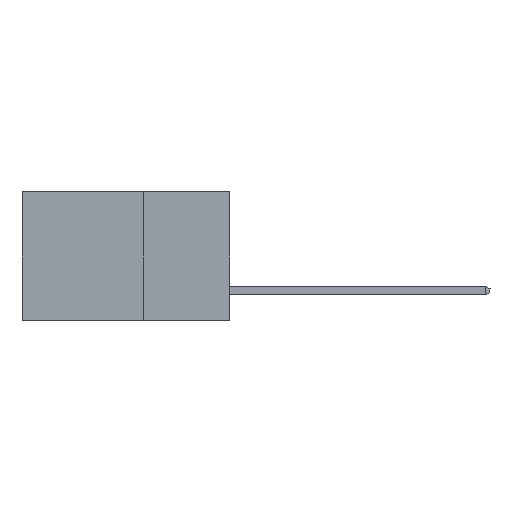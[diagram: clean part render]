
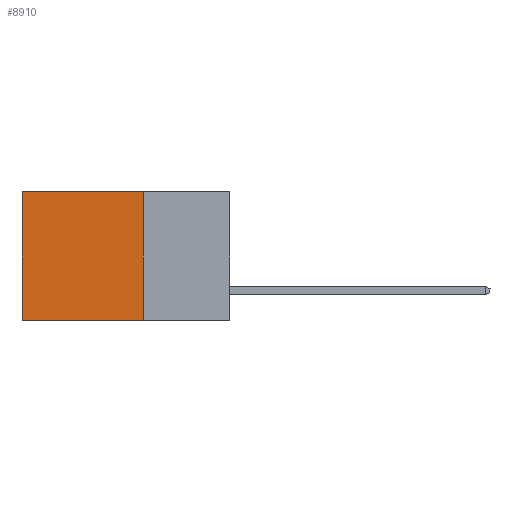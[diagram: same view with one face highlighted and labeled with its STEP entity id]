
A CAD part, left-side view. The second image highlights one B-rep face of the part: STEP entity #8910.
In plain terms, the highlighted planar face has unit normal (-1, 0, 0).
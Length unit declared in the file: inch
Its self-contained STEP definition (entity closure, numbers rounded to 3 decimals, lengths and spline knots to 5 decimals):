
#572 = CARTESIAN_POINT ( 'NONE',  ( 0.2615, 0.6, -0.37 ) ) ;
#685 = VERTEX_POINT ( 'NONE', #4246 ) ;
#836 = CARTESIAN_POINT ( 'NONE',  ( 0.2615, 0.25, -0.37 ) ) ;
#913 = EDGE_CURVE ( 'NONE', #2880, #7285, #18450, .T. ) ;
#2241 = EDGE_LOOP ( 'NONE', ( #13702, #8557, #10275, #5009 ) ) ;
#2442 = CARTESIAN_POINT ( 'NONE',  ( 0.2615, 0.25, 0. ) ) ;
#2776 = CARTESIAN_POINT ( 'NONE',  ( 0.2615, 0.25, -0.37 ) ) ;
#2880 = VERTEX_POINT ( 'NONE', #4384 ) ;
#3271 = VECTOR ( 'NONE', #8469, 39.37008 ) ;
#3718 = DIRECTION ( 'NONE',  ( 1., 0., 0. ) ) ;
#4246 = CARTESIAN_POINT ( 'NONE',  ( 0.2615, 0.25, 0. ) ) ;
#4384 = CARTESIAN_POINT ( 'NONE',  ( 0.2615, 0.6, 0. ) ) ;
#4489 = CARTESIAN_POINT ( 'NONE',  ( 0.2615, 0.25, -0.37 ) ) ;
#5009 = ORIENTED_EDGE ( 'NONE', *, *, #9443, .T. ) ;
#6239 = PLANE ( 'NONE',  #17758 ) ;
#6809 = DIRECTION ( 'NONE',  ( 0., 1., 0. ) ) ;
#6976 = LINE ( 'NONE', #4489, #10486 ) ;
#7156 = CARTESIAN_POINT ( 'NONE',  ( 0.2615, 0.6, -0.37 ) ) ;
#7285 = VERTEX_POINT ( 'NONE', #7156 ) ;
#8469 = DIRECTION ( 'NONE',  ( 0., 0., -1. ) ) ;
#8557 = ORIENTED_EDGE ( 'NONE', *, *, #13276, .F. ) ;
#8822 = LINE ( 'NONE', #10230, #3271 ) ;
#8910 = ADVANCED_FACE ( 'NONE', ( #15175 ), #6239, .F. ) ;
#9443 = EDGE_CURVE ( 'NONE', #685, #2880, #15723, .T. ) ;
#9933 = EDGE_CURVE ( 'NONE', #685, #11783, #8822, .T. ) ;
#10173 = VECTOR ( 'NONE', #6809, 39.37008 ) ;
#10230 = CARTESIAN_POINT ( 'NONE',  ( 0.2615, 0.25, -0.37 ) ) ;
#10275 = ORIENTED_EDGE ( 'NONE', *, *, #9933, .F. ) ;
#10486 = VECTOR ( 'NONE', #16046, 39.37008 ) ;
#11783 = VERTEX_POINT ( 'NONE', #2776 ) ;
#13276 = EDGE_CURVE ( 'NONE', #11783, #7285, #6976, .T. ) ;
#13702 = ORIENTED_EDGE ( 'NONE', *, *, #913, .T. ) ;
#14232 = DIRECTION ( 'NONE',  ( 0., 0., -1. ) ) ;
#15175 = FACE_OUTER_BOUND ( 'NONE', #2241, .T. ) ;
#15723 = LINE ( 'NONE', #2442, #10173 ) ;
#16046 = DIRECTION ( 'NONE',  ( 0., 1., 0. ) ) ;
#16608 = DIRECTION ( 'NONE',  ( 0., 0., -1. ) ) ;
#17314 = VECTOR ( 'NONE', #14232, 39.37008 ) ;
#17758 = AXIS2_PLACEMENT_3D ( 'NONE', #836, #3718, #16608 ) ;
#18450 = LINE ( 'NONE', #572, #17314 ) ;
